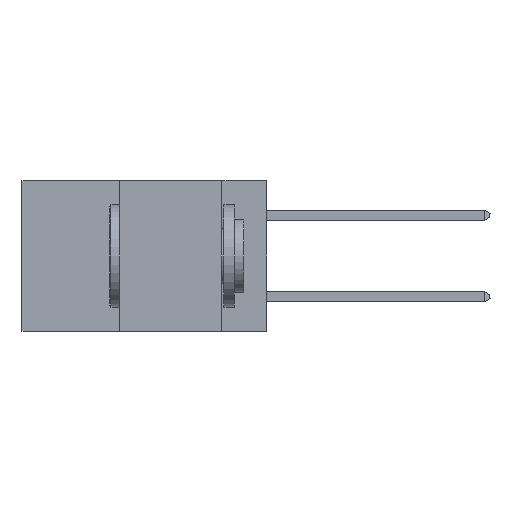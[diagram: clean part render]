
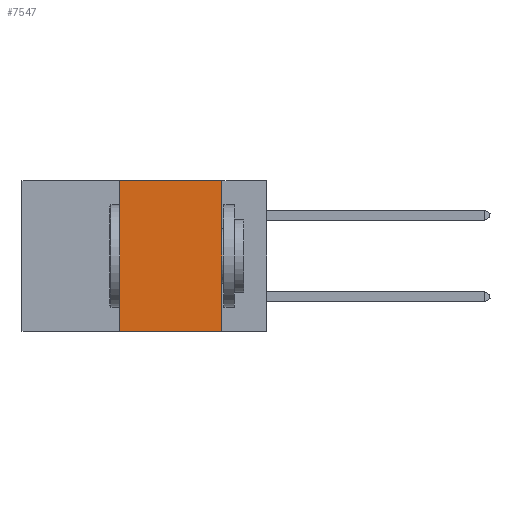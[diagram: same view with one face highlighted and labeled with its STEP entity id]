
A CAD part, left-side view. The second image highlights one B-rep face of the part: STEP entity #7547.
In plain terms, the highlighted planar face has unit normal (-1, 0, 0).
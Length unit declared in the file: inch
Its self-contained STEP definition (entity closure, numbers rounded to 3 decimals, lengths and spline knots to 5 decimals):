
#325 = LINE ( 'NONE', #10844, #13596 ) ;
#1122 = EDGE_CURVE ( 'NONE', #6075, #11867, #9945, .T. ) ;
#1564 = CARTESIAN_POINT ( 'NONE',  ( 0., 0.11, 0. ) ) ;
#2119 = CARTESIAN_POINT ( 'NONE',  ( 0., 0.36, 0. ) ) ;
#2480 = DIRECTION ( 'NONE',  ( 0., -1., 0. ) ) ;
#2512 = VECTOR ( 'NONE', #7137, 39.37008 ) ;
#2853 = EDGE_LOOP ( 'NONE', ( #8832, #12051, #7093, #4924 ) ) ;
#3592 = EDGE_CURVE ( 'NONE', #13428, #6075, #325, .T. ) ;
#4924 = ORIENTED_EDGE ( 'NONE', *, *, #8010, .T. ) ;
#5163 = LINE ( 'NONE', #13081, #2512 ) ;
#5251 = LINE ( 'NONE', #12903, #10645 ) ;
#5303 = DIRECTION ( 'NONE',  ( 1., 0., 0. ) ) ;
#5465 = EDGE_CURVE ( 'NONE', #11867, #9258, #5251, .T. ) ;
#6075 = VERTEX_POINT ( 'NONE', #2119 ) ;
#6173 = FACE_OUTER_BOUND ( 'NONE', #2853, .T. ) ;
#6916 = CARTESIAN_POINT ( 'NONE',  ( 0., 0.36, -0.37 ) ) ;
#7093 = ORIENTED_EDGE ( 'NONE', *, *, #3592, .F. ) ;
#7137 = DIRECTION ( 'NONE',  ( 0., -1., 0. ) ) ;
#7547 = ADVANCED_FACE ( 'NONE', ( #6173 ), #8383, .F. ) ;
#8010 = EDGE_CURVE ( 'NONE', #13428, #9258, #5163, .T. ) ;
#8383 = PLANE ( 'NONE',  #13291 ) ;
#8832 = ORIENTED_EDGE ( 'NONE', *, *, #5465, .F. ) ;
#8853 = CARTESIAN_POINT ( 'NONE',  ( 0., 0.6, 0. ) ) ;
#9258 = VERTEX_POINT ( 'NONE', #9823 ) ;
#9642 = VECTOR ( 'NONE', #2480, 39.37008 ) ;
#9823 = CARTESIAN_POINT ( 'NONE',  ( 0., 0.11, -0.37 ) ) ;
#9945 = LINE ( 'NONE', #8853, #9642 ) ;
#10645 = VECTOR ( 'NONE', #12689, 39.37008 ) ;
#10844 = CARTESIAN_POINT ( 'NONE',  ( 0., 0.36, 0. ) ) ;
#11136 = DIRECTION ( 'NONE',  ( 0., 0., 1. ) ) ;
#11338 = CARTESIAN_POINT ( 'NONE',  ( 0., 0.6, 0. ) ) ;
#11867 = VERTEX_POINT ( 'NONE', #1564 ) ;
#12051 = ORIENTED_EDGE ( 'NONE', *, *, #1122, .F. ) ;
#12348 = DIRECTION ( 'NONE',  ( 0., 0., -1. ) ) ;
#12689 = DIRECTION ( 'NONE',  ( 0., 0., -1. ) ) ;
#12903 = CARTESIAN_POINT ( 'NONE',  ( 0., 0.11, 0. ) ) ;
#13081 = CARTESIAN_POINT ( 'NONE',  ( 0., 0.6, -0.37 ) ) ;
#13291 = AXIS2_PLACEMENT_3D ( 'NONE', #11338, #5303, #12348 ) ;
#13428 = VERTEX_POINT ( 'NONE', #6916 ) ;
#13596 = VECTOR ( 'NONE', #11136, 39.37008 ) ;
